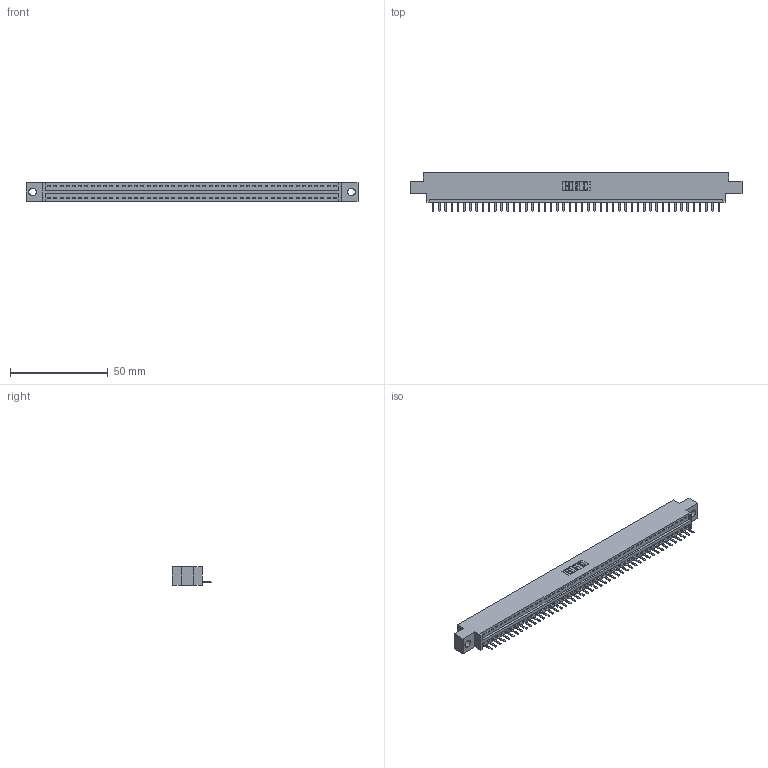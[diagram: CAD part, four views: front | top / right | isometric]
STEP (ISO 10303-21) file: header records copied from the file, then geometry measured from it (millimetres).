
FILE_DESCRIPTION (( 'STEP AP203' ), '1' );
FILE_NAME ('346-047-520-604.STEP', '2022-05-09T21:15:34', ( '' ), ( '' ), 'SwSTEP 2.0', 'SolidWorks 2020', '' );
FILE_SCHEMA (( 'CONFIG_CONTROL_DESIGN' ));
Length unit declared in the file: inch
Products named in the file (3): 346-047-520-604; 345-292-001_345-293-120; 346 Part_0.170 Offset - 0.156 Dia-TH
Assembly tree (48 placements, depth 2):
  346-047-520-604
    346 Part_0.170 Offset - 0.156 Dia-TH
    345-292-001_345-293-120  x47
Bounding box: 169.8 x 20.02 x 9.4 mm (x, y, z)
Volume: 15892.2 mm3; surface area: 19463.5 mm2
Topology: 48 solids, 48 shells, 3054 faces, 9025 edges, 5890 vertices
Faces by surface type: plane 2068, cylinder 986
Entity records: 29161 total; most frequent: CARTESIAN_POINT 5019, ORIENTED_EDGE 4986, DIRECTION 4407, EDGE_CURVE 2493, VECTOR 2169, LINE 2169, VERTEX_POINT 1658, AXIS2_PLACEMENT_3D 1119
